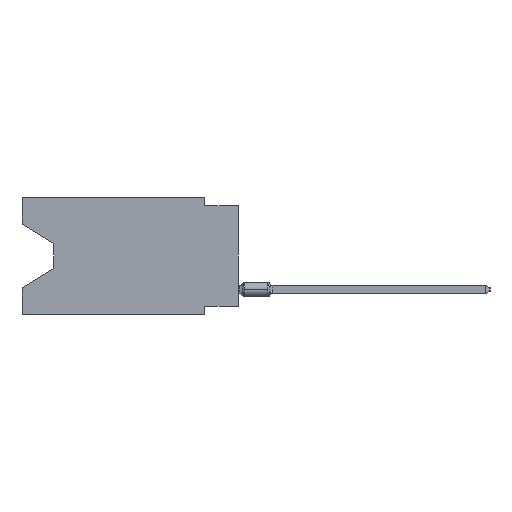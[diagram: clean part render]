
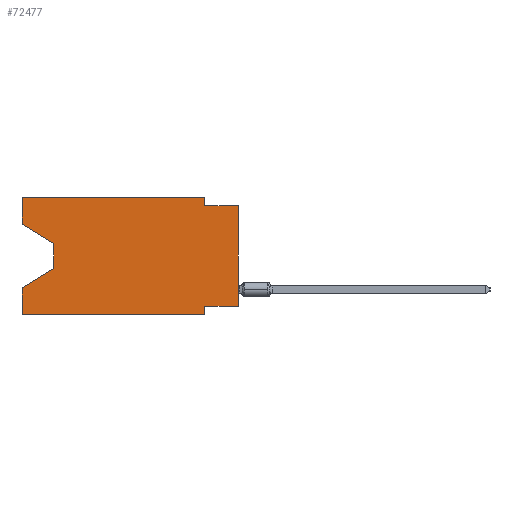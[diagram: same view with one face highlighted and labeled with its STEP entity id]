
A CAD part, left-side view. The second image highlights one B-rep face of the part: STEP entity #72477.
In plain terms, the highlighted planar face has unit normal (-1, 0, 0).
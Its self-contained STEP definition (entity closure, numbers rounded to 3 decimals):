
#333 = DIRECTION ( 'NONE',  ( 0., 0., 1. ) ) ;
#1187 = CARTESIAN_POINT ( 'NONE',  ( 0., 13.97, -5.385 ) ) ;
#1813 = ORIENTED_EDGE ( 'NONE', *, *, #10173, .F. ) ;
#2568 = LINE ( 'NONE', #40262, #28659 ) ;
#3293 = ORIENTED_EDGE ( 'NONE', *, *, #33610, .T. ) ;
#4296 = ORIENTED_EDGE ( 'NONE', *, *, #55824, .F. ) ;
#4357 = EDGE_CURVE ( 'NONE', #66656, #15986, #19547, .T. ) ;
#4408 = CARTESIAN_POINT ( 'NONE',  ( 0., 16.383, 0. ) ) ;
#4839 = EDGE_LOOP ( 'NONE', ( #50200, #3293, #15315, #65770, #21620, #15379, #4296, #17349, #1813, #38132, #53108, #78437 ) ) ;
#4969 = DIRECTION ( 'NONE',  ( 0., 0., -1. ) ) ;
#5726 = VERTEX_POINT ( 'NONE', #59203 ) ;
#5801 = VECTOR ( 'NONE', #10001, 1000. ) ;
#6673 = LINE ( 'NONE', #4408, #36608 ) ;
#8545 = VERTEX_POINT ( 'NONE', #59087 ) ;
#8598 = EDGE_CURVE ( 'NONE', #65358, #57113, #36059, .T. ) ;
#9307 = CARTESIAN_POINT ( 'NONE',  ( 0., 16.383, -2.038 ) ) ;
#9526 = VERTEX_POINT ( 'NONE', #61527 ) ;
#9668 = DIRECTION ( 'NONE',  ( 0., 1., 0. ) ) ;
#10001 = DIRECTION ( 'NONE',  ( 0., 0., 1. ) ) ;
#10173 = EDGE_CURVE ( 'NONE', #36186, #14916, #24080, .T. ) ;
#10240 = CARTESIAN_POINT ( 'NONE',  ( 0., 0., -0.635 ) ) ;
#11755 = DIRECTION ( 'NONE',  ( 0., -1., 0. ) ) ;
#12272 = EDGE_CURVE ( 'NONE', #57113, #8545, #6673, .T. ) ;
#13622 = DIRECTION ( 'NONE',  ( 0., 0., -1. ) ) ;
#14916 = VERTEX_POINT ( 'NONE', #10240 ) ;
#15315 = ORIENTED_EDGE ( 'NONE', *, *, #4357, .T. ) ;
#15379 = ORIENTED_EDGE ( 'NONE', *, *, #64913, .F. ) ;
#15986 = VERTEX_POINT ( 'NONE', #22593 ) ;
#17185 = VECTOR ( 'NONE', #18802, 1000. ) ;
#17349 = ORIENTED_EDGE ( 'NONE', *, *, #33882, .T. ) ;
#18802 = DIRECTION ( 'NONE',  ( 0., 0., 1. ) ) ;
#19270 = VECTOR ( 'NONE', #57391, 1000. ) ;
#19425 = EDGE_CURVE ( 'NONE', #9526, #5726, #65395, .T. ) ;
#19547 = LINE ( 'NONE', #43777, #67407 ) ;
#19948 = VECTOR ( 'NONE', #11755, 1000. ) ;
#20145 = CARTESIAN_POINT ( 'NONE',  ( 0., 16.383, 0. ) ) ;
#20530 = CARTESIAN_POINT ( 'NONE',  ( 0., 0., -8.255 ) ) ;
#21620 = ORIENTED_EDGE ( 'NONE', *, *, #19425, .T. ) ;
#21715 = DIRECTION ( 'NONE',  ( 0., 0., -1. ) ) ;
#22105 = LINE ( 'NONE', #53457, #74852 ) ;
#22593 = CARTESIAN_POINT ( 'NONE',  ( 0., 16.383, -6.852 ) ) ;
#24080 = LINE ( 'NONE', #29243, #19948 ) ;
#28659 = VECTOR ( 'NONE', #9668, 1000. ) ;
#29072 = AXIS2_PLACEMENT_3D ( 'NONE', #20145, #62984, #38019 ) ;
#29243 = CARTESIAN_POINT ( 'NONE',  ( 0., 0., -0.635 ) ) ;
#30404 = EDGE_CURVE ( 'NONE', #65358, #57750, #33193, .T. ) ;
#30470 = EDGE_CURVE ( 'NONE', #8545, #36186, #47435, .T. ) ;
#33193 = LINE ( 'NONE', #39532, #19270 ) ;
#33610 = EDGE_CURVE ( 'NONE', #57750, #66656, #68002, .T. ) ;
#33873 = CARTESIAN_POINT ( 'NONE',  ( 0., 2.54, -0.635 ) ) ;
#33882 = EDGE_CURVE ( 'NONE', #68324, #14916, #52489, .T. ) ;
#35651 = DIRECTION ( 'NONE',  ( 0., -1., 0. ) ) ;
#36059 = LINE ( 'NONE', #60257, #42755 ) ;
#36186 = VERTEX_POINT ( 'NONE', #33873 ) ;
#36608 = VECTOR ( 'NONE', #55090, 1000. ) ;
#37464 = VECTOR ( 'NONE', #35651, 1000. ) ;
#37630 = FACE_OUTER_BOUND ( 'NONE', #4839, .T. ) ;
#37866 = CARTESIAN_POINT ( 'NONE',  ( 0., 16.383, 0. ) ) ;
#38019 = DIRECTION ( 'NONE',  ( 0., 0., -1. ) ) ;
#38132 = ORIENTED_EDGE ( 'NONE', *, *, #30470, .F. ) ;
#39310 = LINE ( 'NONE', #37866, #17185 ) ;
#39532 = CARTESIAN_POINT ( 'NONE',  ( 0., 16.383, -2.038 ) ) ;
#39767 = CARTESIAN_POINT ( 'NONE',  ( 0., 2.54, -8.255 ) ) ;
#40262 = CARTESIAN_POINT ( 'NONE',  ( 0., 0., -8.255 ) ) ;
#40879 = VECTOR ( 'NONE', #4969, 1000. ) ;
#42755 = VECTOR ( 'NONE', #333, 1000. ) ;
#43777 = CARTESIAN_POINT ( 'NONE',  ( 0., 13.97, -5.385 ) ) ;
#46546 = CARTESIAN_POINT ( 'NONE',  ( 0., 0., 0. ) ) ;
#47046 = CARTESIAN_POINT ( 'NONE',  ( 0., 2.54, 0. ) ) ;
#47435 = LINE ( 'NONE', #47046, #40879 ) ;
#48970 = CARTESIAN_POINT ( 'NONE',  ( 0., 13.97, -3.505 ) ) ;
#50200 = ORIENTED_EDGE ( 'NONE', *, *, #30404, .T. ) ;
#50322 = PLANE ( 'NONE',  #29072 ) ;
#50356 = VECTOR ( 'NONE', #13622, 1000. ) ;
#50440 = CARTESIAN_POINT ( 'NONE',  ( 0., 13.97, -3.505 ) ) ;
#52489 = LINE ( 'NONE', #46546, #5801 ) ;
#53108 = ORIENTED_EDGE ( 'NONE', *, *, #12272, .F. ) ;
#53457 = CARTESIAN_POINT ( 'NONE',  ( 0., 2.54, -8.89 ) ) ;
#55090 = DIRECTION ( 'NONE',  ( 0., -1., 0. ) ) ;
#55824 = EDGE_CURVE ( 'NONE', #68324, #56378, #2568, .T. ) ;
#56378 = VERTEX_POINT ( 'NONE', #39767 ) ;
#57113 = VERTEX_POINT ( 'NONE', #74528 ) ;
#57391 = DIRECTION ( 'NONE',  ( 0., -0.855, -0.519 ) ) ;
#57750 = VERTEX_POINT ( 'NONE', #50440 ) ;
#59040 = EDGE_CURVE ( 'NONE', #9526, #15986, #39310, .T. ) ;
#59087 = CARTESIAN_POINT ( 'NONE',  ( 0., 2.54, 0. ) ) ;
#59203 = CARTESIAN_POINT ( 'NONE',  ( 0., 2.54, -8.89 ) ) ;
#60257 = CARTESIAN_POINT ( 'NONE',  ( 0., 16.383, 0. ) ) ;
#61527 = CARTESIAN_POINT ( 'NONE',  ( 0., 16.383, -8.89 ) ) ;
#62777 = DIRECTION ( 'NONE',  ( 0., 0.855, -0.519 ) ) ;
#62984 = DIRECTION ( 'NONE',  ( 1., 0., 0. ) ) ;
#64913 = EDGE_CURVE ( 'NONE', #56378, #5726, #22105, .T. ) ;
#65358 = VERTEX_POINT ( 'NONE', #9307 ) ;
#65395 = LINE ( 'NONE', #71357, #37464 ) ;
#65770 = ORIENTED_EDGE ( 'NONE', *, *, #59040, .F. ) ;
#66656 = VERTEX_POINT ( 'NONE', #1187 ) ;
#67407 = VECTOR ( 'NONE', #62777, 1000. ) ;
#68002 = LINE ( 'NONE', #48970, #50356 ) ;
#68324 = VERTEX_POINT ( 'NONE', #20530 ) ;
#71357 = CARTESIAN_POINT ( 'NONE',  ( 0., 16.383, -8.89 ) ) ;
#72477 = ADVANCED_FACE ( 'NONE', ( #37630 ), #50322, .F. ) ;
#74528 = CARTESIAN_POINT ( 'NONE',  ( 0., 16.383, 0. ) ) ;
#74852 = VECTOR ( 'NONE', #21715, 1000. ) ;
#78437 = ORIENTED_EDGE ( 'NONE', *, *, #8598, .F. ) ;
